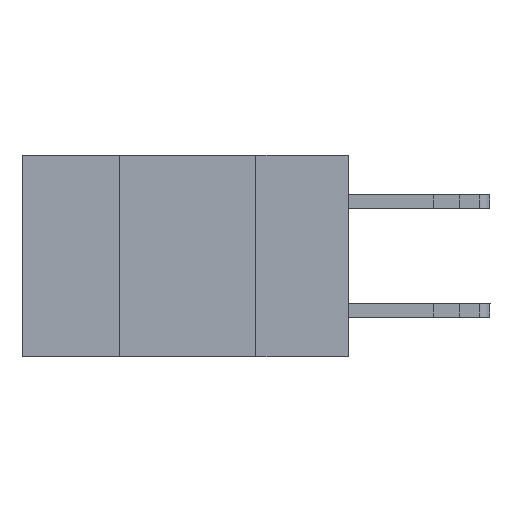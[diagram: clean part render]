
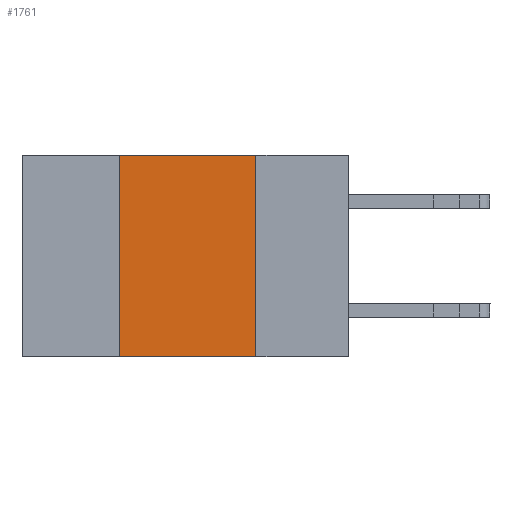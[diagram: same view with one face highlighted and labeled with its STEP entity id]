
A CAD part, left-side view. The second image highlights one B-rep face of the part: STEP entity #1761.
In plain terms, the highlighted planar face has unit normal (-1, 0, 0).
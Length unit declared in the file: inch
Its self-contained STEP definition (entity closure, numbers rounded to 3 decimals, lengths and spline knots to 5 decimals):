
#889 = VERTEX_POINT ( 'NONE', #1948 ) ;
#1151 = DIRECTION ( 'NONE',  ( 0., 0., 1. ) ) ;
#1224 = VERTEX_POINT ( 'NONE', #11138 ) ;
#1321 = CARTESIAN_POINT ( 'NONE',  ( 0., 0.17, -0.37 ) ) ;
#1761 = ADVANCED_FACE ( 'NONE', ( #6393 ), #8048, .F. ) ;
#1948 = CARTESIAN_POINT ( 'NONE',  ( 0., 0.42, -0.37 ) ) ;
#2876 = DIRECTION ( 'NONE',  ( 0., 0., -1. ) ) ;
#3339 = CARTESIAN_POINT ( 'NONE',  ( 0., 0.42, 0. ) ) ;
#3568 = CARTESIAN_POINT ( 'NONE',  ( 0., 0.17, -0.37 ) ) ;
#3793 = LINE ( 'NONE', #5655, #13619 ) ;
#4209 = CARTESIAN_POINT ( 'NONE',  ( 0., 0.6, -0.37 ) ) ;
#5026 = ORIENTED_EDGE ( 'NONE', *, *, #14553, .F. ) ;
#5610 = DIRECTION ( 'NONE',  ( 0., -1., 0. ) ) ;
#5655 = CARTESIAN_POINT ( 'NONE',  ( 0., 0.6, 0. ) ) ;
#5793 = ORIENTED_EDGE ( 'NONE', *, *, #16204, .F. ) ;
#6391 = VECTOR ( 'NONE', #1151, 39.37008 ) ;
#6393 = FACE_OUTER_BOUND ( 'NONE', #11116, .T. ) ;
#6575 = VECTOR ( 'NONE', #5610, 39.37008 ) ;
#7021 = DIRECTION ( 'NONE',  ( 0., -1., 0. ) ) ;
#7501 = VECTOR ( 'NONE', #2876, 39.37008 ) ;
#7825 = LINE ( 'NONE', #4209, #6575 ) ;
#7846 = DIRECTION ( 'NONE',  ( 0., 0., -1. ) ) ;
#7864 = DIRECTION ( 'NONE',  ( 1., 0., 0. ) ) ;
#7916 = CARTESIAN_POINT ( 'NONE',  ( 0., 0.6, 0. ) ) ;
#8048 = PLANE ( 'NONE',  #9070 ) ;
#9070 = AXIS2_PLACEMENT_3D ( 'NONE', #7916, #7864, #7846 ) ;
#9470 = LINE ( 'NONE', #17209, #6391 ) ;
#11028 = LINE ( 'NONE', #1321, #7501 ) ;
#11116 = EDGE_LOOP ( 'NONE', ( #5026, #15237, #5793, #13499 ) ) ;
#11138 = CARTESIAN_POINT ( 'NONE',  ( 0., 0.17, 0. ) ) ;
#13499 = ORIENTED_EDGE ( 'NONE', *, *, #17030, .T. ) ;
#13619 = VECTOR ( 'NONE', #7021, 39.37008 ) ;
#14081 = VERTEX_POINT ( 'NONE', #3339 ) ;
#14553 = EDGE_CURVE ( 'NONE', #1224, #14968, #11028, .T. ) ;
#14968 = VERTEX_POINT ( 'NONE', #3568 ) ;
#15237 = ORIENTED_EDGE ( 'NONE', *, *, #15400, .F. ) ;
#15400 = EDGE_CURVE ( 'NONE', #14081, #1224, #3793, .T. ) ;
#16204 = EDGE_CURVE ( 'NONE', #889, #14081, #9470, .T. ) ;
#17030 = EDGE_CURVE ( 'NONE', #889, #14968, #7825, .T. ) ;
#17209 = CARTESIAN_POINT ( 'NONE',  ( 0., 0.42, -0.37 ) ) ;
